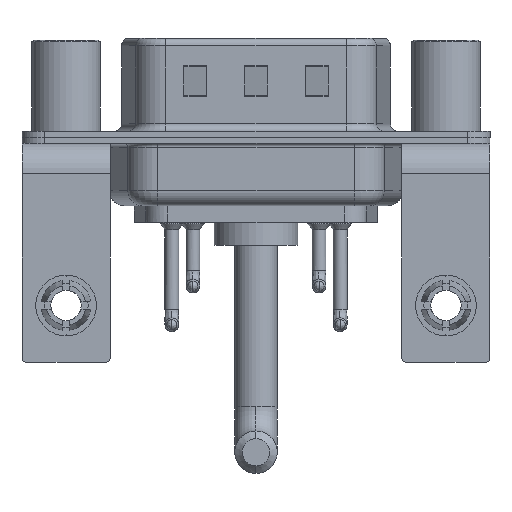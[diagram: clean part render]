
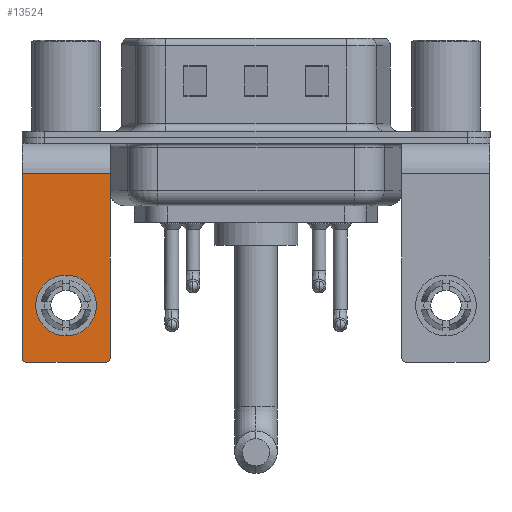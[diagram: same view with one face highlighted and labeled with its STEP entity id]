
A CAD part, front view. The second image highlights one B-rep face of the part: STEP entity #13524.
In plain terms, the highlighted planar face has unit normal (0, -1, 0).
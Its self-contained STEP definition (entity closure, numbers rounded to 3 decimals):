
#130 = DIRECTION ( 'NONE',  ( 0., 0., 1. ) ) ;
#354 = ORIENTED_EDGE ( 'NONE', *, *, #13753, .T. ) ;
#792 = VERTEX_POINT ( 'NONE', #13446 ) ;
#977 = LINE ( 'NONE', #2755, #19424 ) ;
#1027 = ORIENTED_EDGE ( 'NONE', *, *, #7658, .T. ) ;
#1272 = AXIS2_PLACEMENT_3D ( 'NONE', #4437, #22265, #5980 ) ;
#2153 = VERTEX_POINT ( 'NONE', #13452 ) ;
#2276 = CARTESIAN_POINT ( 'NONE',  ( 0., -6.25, -9.07 ) ) ;
#2626 = CARTESIAN_POINT ( 'NONE',  ( -2.9, -6.25, -2.4 ) ) ;
#2755 = CARTESIAN_POINT ( 'NONE',  ( 2.9, -6.25, -2.4 ) ) ;
#2915 = EDGE_CURVE ( 'NONE', #19599, #19192, #17529, .T. ) ;
#2999 = VECTOR ( 'NONE', #14318, 1000. ) ;
#3940 = DIRECTION ( 'NONE',  ( -1., 0., 0. ) ) ;
#4163 = EDGE_CURVE ( 'NONE', #21169, #2153, #977, .T. ) ;
#4437 = CARTESIAN_POINT ( 'NONE',  ( 2.65, -6.25, -14.55 ) ) ;
#4905 = CARTESIAN_POINT ( 'NONE',  ( 2.9, -6.25, -2.4 ) ) ;
#5336 = DIRECTION ( 'NONE',  ( 0., 1., 0. ) ) ;
#5980 = DIRECTION ( 'NONE',  ( 0., 0., 1. ) ) ;
#7247 = AXIS2_PLACEMENT_3D ( 'NONE', #19323, #15404, #8246 ) ;
#7658 = EDGE_CURVE ( 'NONE', #13819, #2153, #16474, .T. ) ;
#8163 = ORIENTED_EDGE ( 'NONE', *, *, #20897, .T. ) ;
#8246 = DIRECTION ( 'NONE',  ( 0., 0., 1. ) ) ;
#8252 = AXIS2_PLACEMENT_3D ( 'NONE', #14162, #21392, #130 ) ;
#8554 = ORIENTED_EDGE ( 'NONE', *, *, #13052, .F. ) ;
#9683 = CARTESIAN_POINT ( 'NONE',  ( -2.9, -6.25, -14.55 ) ) ;
#10008 = VECTOR ( 'NONE', #11374, 1000. ) ;
#10444 = DIRECTION ( 'NONE',  ( 0., 0., 1. ) ) ;
#11239 = CIRCLE ( 'NONE', #23005, 2. ) ;
#11374 = DIRECTION ( 'NONE',  ( 0., 0., -1. ) ) ;
#11411 = CARTESIAN_POINT ( 'NONE',  ( 2.65, -6.25, -14.8 ) ) ;
#12499 = CIRCLE ( 'NONE', #17817, 2. ) ;
#12964 = EDGE_LOOP ( 'NONE', ( #23051, #19120, #8554, #1027, #15141, #14654 ) ) ;
#12979 = CARTESIAN_POINT ( 'NONE',  ( -2.65, -6.25, -14.8 ) ) ;
#13052 = EDGE_CURVE ( 'NONE', #13819, #19192, #16345, .T. ) ;
#13350 = DIRECTION ( 'NONE',  ( 0., 0., -1. ) ) ;
#13430 = CARTESIAN_POINT ( 'NONE',  ( 0., -6.25, -11.07 ) ) ;
#13446 = CARTESIAN_POINT ( 'NONE',  ( 0., -6.25, -13.07 ) ) ;
#13452 = CARTESIAN_POINT ( 'NONE',  ( 2.9, -6.25, -14.55 ) ) ;
#13524 = ADVANCED_FACE ( 'NONE', ( #14290, #19979 ), #17857, .F. ) ;
#13753 = EDGE_CURVE ( 'NONE', #14078, #792, #12499, .T. ) ;
#13819 = VERTEX_POINT ( 'NONE', #11411 ) ;
#14078 = VERTEX_POINT ( 'NONE', #2276 ) ;
#14162 = CARTESIAN_POINT ( 'NONE',  ( 2.9, -6.25, -2.4 ) ) ;
#14290 = FACE_BOUND ( 'NONE', #16239, .T. ) ;
#14318 = DIRECTION ( 'NONE',  ( -1., 0., 0. ) ) ;
#14654 = ORIENTED_EDGE ( 'NONE', *, *, #19194, .T. ) ;
#15103 = DIRECTION ( 'NONE',  ( 0., 1., 0. ) ) ;
#15111 = LINE ( 'NONE', #16428, #16497 ) ;
#15141 = ORIENTED_EDGE ( 'NONE', *, *, #4163, .F. ) ;
#15404 = DIRECTION ( 'NONE',  ( 0., -1., 0. ) ) ;
#16239 = EDGE_LOOP ( 'NONE', ( #8163, #354 ) ) ;
#16345 = LINE ( 'NONE', #23447, #2999 ) ;
#16428 = CARTESIAN_POINT ( 'NONE',  ( 2.9, -6.25, -2.4 ) ) ;
#16474 = CIRCLE ( 'NONE', #1272, 0.25 ) ;
#16497 = VECTOR ( 'NONE', #3940, 1000. ) ;
#16539 = DIRECTION ( 'NONE',  ( 0., 0., 1. ) ) ;
#17356 = EDGE_CURVE ( 'NONE', #18104, #19599, #20525, .T. ) ;
#17529 = CIRCLE ( 'NONE', #7247, 0.25 ) ;
#17817 = AXIS2_PLACEMENT_3D ( 'NONE', #13430, #15103, #16539 ) ;
#17857 = PLANE ( 'NONE',  #8252 ) ;
#18104 = VERTEX_POINT ( 'NONE', #2626 ) ;
#19120 = ORIENTED_EDGE ( 'NONE', *, *, #2915, .T. ) ;
#19192 = VERTEX_POINT ( 'NONE', #12979 ) ;
#19194 = EDGE_CURVE ( 'NONE', #21169, #18104, #15111, .T. ) ;
#19323 = CARTESIAN_POINT ( 'NONE',  ( -2.65, -6.25, -14.55 ) ) ;
#19424 = VECTOR ( 'NONE', #13350, 1000. ) ;
#19599 = VERTEX_POINT ( 'NONE', #9683 ) ;
#19979 = FACE_OUTER_BOUND ( 'NONE', #12964, .T. ) ;
#20171 = CARTESIAN_POINT ( 'NONE',  ( -2.9, -6.25, -2.4 ) ) ;
#20525 = LINE ( 'NONE', #20171, #10008 ) ;
#20897 = EDGE_CURVE ( 'NONE', #792, #14078, #11239, .T. ) ;
#21169 = VERTEX_POINT ( 'NONE', #4905 ) ;
#21392 = DIRECTION ( 'NONE',  ( 0., 1., 0. ) ) ;
#21498 = CARTESIAN_POINT ( 'NONE',  ( 0., -6.25, -11.07 ) ) ;
#22265 = DIRECTION ( 'NONE',  ( 0., -1., 0. ) ) ;
#23005 = AXIS2_PLACEMENT_3D ( 'NONE', #21498, #5336, #10444 ) ;
#23051 = ORIENTED_EDGE ( 'NONE', *, *, #17356, .T. ) ;
#23447 = CARTESIAN_POINT ( 'NONE',  ( 2.9, -6.25, -14.8 ) ) ;
